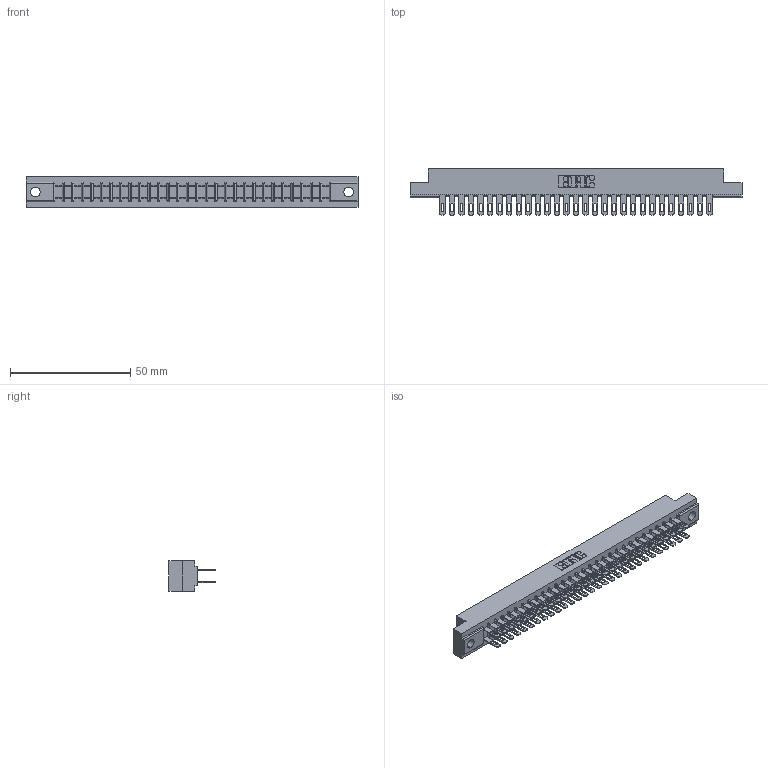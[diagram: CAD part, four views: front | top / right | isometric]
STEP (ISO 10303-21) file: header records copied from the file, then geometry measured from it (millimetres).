
FILE_DESCRIPTION (( 'STEP AP203' ), '1' );
FILE_NAME ('307-058-400-204.STEP', '2020-09-30T11:40:48', ( '' ), ( '' ), 'SwSTEP 2.0', 'SolidWorks 2020', '' );
FILE_SCHEMA (( 'CONFIG_CONTROL_DESIGN' ));
Length unit declared in the file: inch
Products named in the file (3): 307-058-400-204; 307-290-001_500; 307 Part_.156 Dia Mounting Holes
Assembly tree (59 placements, depth 2):
  307-058-400-204
    307 Part_.156 Dia Mounting Holes
    307-290-001_500  x58
Bounding box: 137.92 x 19.18 x 12.7 mm (x, y, z)
Volume: 14634.5 mm3; surface area: 18400.2 mm2
Topology: 59 solids, 59 shells, 2830 faces, 7899 edges, 5106 vertices
Faces by surface type: plane 1824, cylinder 946, sphere 60
Entity records: 27784 total; most frequent: CARTESIAN_POINT 4551, ORIENTED_EDGE 4506, DIRECTION 4457, EDGE_CURVE 2253, LINE 1729, VECTOR 1729, VERTEX_POINT 1458, AXIS2_PLACEMENT_3D 1364
